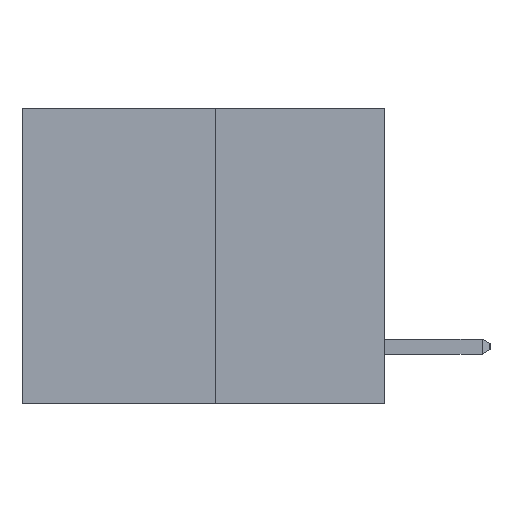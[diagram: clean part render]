
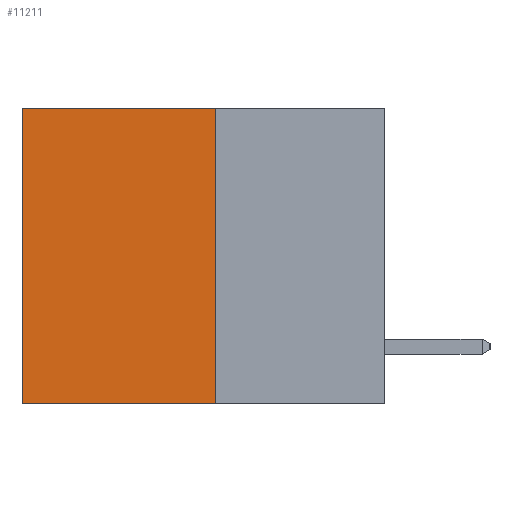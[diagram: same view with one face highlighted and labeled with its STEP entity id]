
A CAD part, left-side view. The second image highlights one B-rep face of the part: STEP entity #11211.
In plain terms, the highlighted planar face has unit normal (-1, 0, 0).
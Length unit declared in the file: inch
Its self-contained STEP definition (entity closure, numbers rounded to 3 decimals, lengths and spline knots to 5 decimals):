
#68 = FACE_OUTER_BOUND ( 'NONE', #21718, .T. ) ;
#100 = VERTEX_POINT ( 'NONE', #9641 ) ;
#2414 = DIRECTION ( 'NONE',  ( 1., 0., 0. ) ) ;
#3691 = VERTEX_POINT ( 'NONE', #8992 ) ;
#6072 = AXIS2_PLACEMENT_3D ( 'NONE', #20795, #2414, #18887 ) ;
#6302 = ORIENTED_EDGE ( 'NONE', *, *, #7756, .T. ) ;
#6749 = CARTESIAN_POINT ( 'NONE',  ( 0.3165, 0.28, 0. ) ) ;
#7567 = DIRECTION ( 'NONE',  ( 0., 1., 0. ) ) ;
#7584 = LINE ( 'NONE', #18228, #12386 ) ;
#7756 = EDGE_CURVE ( 'NONE', #11344, #100, #26046, .T. ) ;
#8078 = VERTEX_POINT ( 'NONE', #26666 ) ;
#8992 = CARTESIAN_POINT ( 'NONE',  ( 0.3165, 0.28, 0. ) ) ;
#9641 = CARTESIAN_POINT ( 'NONE',  ( 0.3165, 0.6, -0.49 ) ) ;
#9787 = LINE ( 'NONE', #6749, #24246 ) ;
#10005 = ORIENTED_EDGE ( 'NONE', *, *, #21164, .F. ) ;
#10146 = CARTESIAN_POINT ( 'NONE',  ( 0.3165, 0.6, -0.49 ) ) ;
#10352 = ORIENTED_EDGE ( 'NONE', *, *, #18476, .F. ) ;
#11211 = ADVANCED_FACE ( 'NONE', ( #68 ), #16366, .F. ) ;
#11344 = VERTEX_POINT ( 'NONE', #15174 ) ;
#12068 = DIRECTION ( 'NONE',  ( 0., 0., -1. ) ) ;
#12386 = VECTOR ( 'NONE', #12068, 39.37008 ) ;
#12577 = EDGE_CURVE ( 'NONE', #3691, #11344, #9787, .T. ) ;
#14448 = VECTOR ( 'NONE', #25065, 39.37008 ) ;
#15174 = CARTESIAN_POINT ( 'NONE',  ( 0.3165, 0.6, 0. ) ) ;
#16366 = PLANE ( 'NONE',  #6072 ) ;
#16390 = ORIENTED_EDGE ( 'NONE', *, *, #12577, .T. ) ;
#17932 = CARTESIAN_POINT ( 'NONE',  ( 0.3165, 0.28, -0.49 ) ) ;
#18228 = CARTESIAN_POINT ( 'NONE',  ( 0.3165, 0.28, -0.49 ) ) ;
#18476 = EDGE_CURVE ( 'NONE', #3691, #8078, #7584, .T. ) ;
#18887 = DIRECTION ( 'NONE',  ( 0., 0., -1. ) ) ;
#19658 = VECTOR ( 'NONE', #7567, 39.37008 ) ;
#20795 = CARTESIAN_POINT ( 'NONE',  ( 0.3165, 0.28, -0.49 ) ) ;
#21164 = EDGE_CURVE ( 'NONE', #8078, #100, #24775, .T. ) ;
#21718 = EDGE_LOOP ( 'NONE', ( #6302, #10005, #10352, #16390 ) ) ;
#23011 = DIRECTION ( 'NONE',  ( 0., 1., 0. ) ) ;
#24246 = VECTOR ( 'NONE', #23011, 39.37008 ) ;
#24775 = LINE ( 'NONE', #17932, #19658 ) ;
#25065 = DIRECTION ( 'NONE',  ( 0., 0., -1. ) ) ;
#26046 = LINE ( 'NONE', #10146, #14448 ) ;
#26666 = CARTESIAN_POINT ( 'NONE',  ( 0.3165, 0.28, -0.49 ) ) ;
